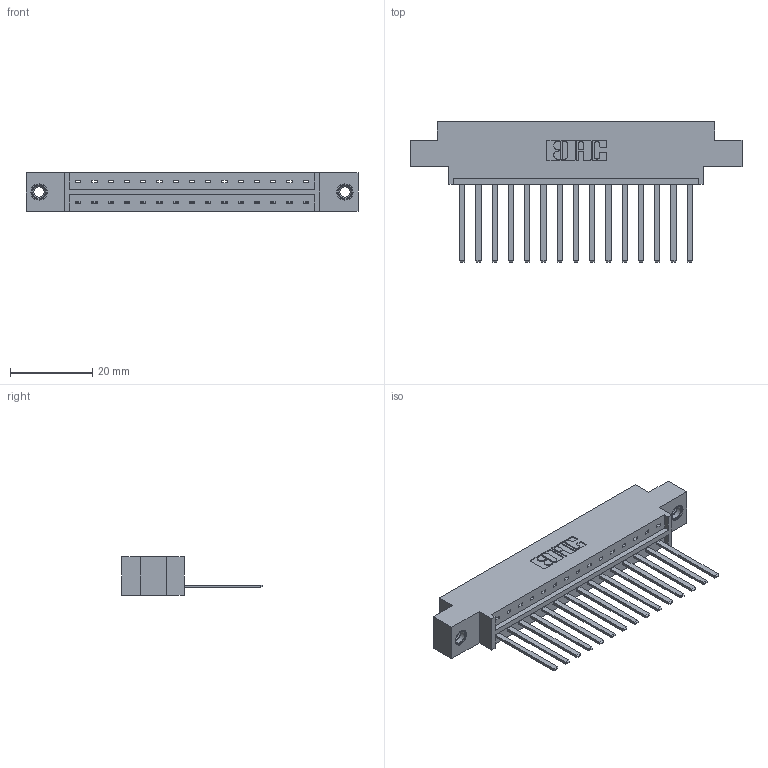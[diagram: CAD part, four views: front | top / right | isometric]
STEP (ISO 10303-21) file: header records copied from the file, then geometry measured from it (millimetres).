
FILE_DESCRIPTION (( 'STEP AP203' ), '1' );
FILE_NAME ('333-015-544-607.STEP', '2018-08-01T04:00:53', ( '' ), ( '' ), 'SwSTEP 2.0', 'SolidWorks 2016', '' );
FILE_SCHEMA (( 'CONFIG_CONTROL_DESIGN' ));
Length unit declared in the file: inch
Products named in the file (4): 345-292-001_345-293-144; 345-250-001_345-250-005-103; 333-015-544-607; 333 Part_Offset - .156 Dia - TI
Assembly tree (18 placements, depth 2):
  333-015-544-607
    333 Part_Offset - .156 Dia - TI
    345-292-001_345-293-144  x15
    345-250-001_345-250-005-103  x2
Bounding box: 80.98 x 34.3 x 9.4 mm (x, y, z)
Volume: 7848.6 mm3; surface area: 9115.7 mm2
Topology: 18 solids, 18 shells, 958 faces, 2829 edges, 1858 vertices
Faces by surface type: plane 676, cylinder 266, cone 12, torus 4
Entity records: 13796 total; most frequent: CARTESIAN_POINT 2366, ORIENTED_EDGE 2310, DIRECTION 2079, EDGE_CURVE 1155, LINE 1011, VECTOR 1011, VERTEX_POINT 764, AXIS2_PLACEMENT_3D 534
